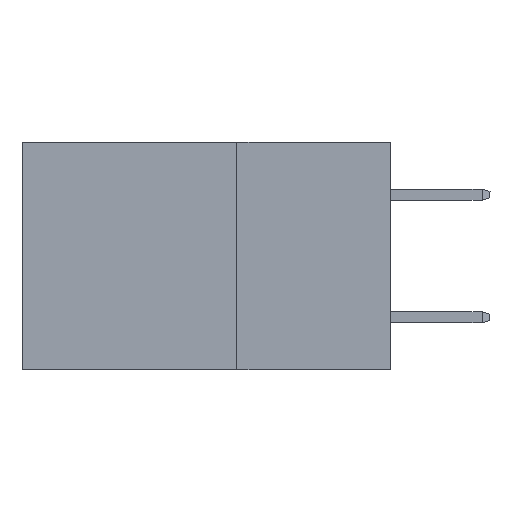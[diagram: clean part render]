
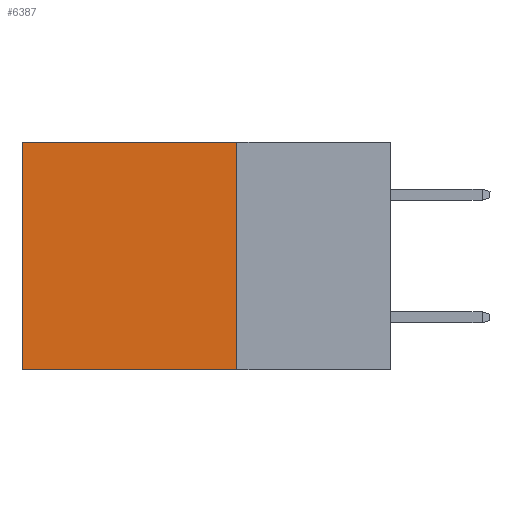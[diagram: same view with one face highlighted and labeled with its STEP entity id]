
A CAD part, left-side view. The second image highlights one B-rep face of the part: STEP entity #6387.
In plain terms, the highlighted planar face has unit normal (-1, 0, 0).
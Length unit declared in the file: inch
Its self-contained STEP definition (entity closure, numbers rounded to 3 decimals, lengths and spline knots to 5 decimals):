
#381 = CARTESIAN_POINT ( 'NONE',  ( 0.2875, 0.25, -0.37 ) ) ;
#484 = EDGE_CURVE ( 'NONE', #5488, #2101, #5989, .T. ) ;
#674 = EDGE_CURVE ( 'NONE', #6831, #8876, #8755, .T. ) ;
#713 = ORIENTED_EDGE ( 'NONE', *, *, #674, .F. ) ;
#784 = LINE ( 'NONE', #3732, #4595 ) ;
#889 = CARTESIAN_POINT ( 'NONE',  ( 0.2875, 0.6, 0. ) ) ;
#1172 = VECTOR ( 'NONE', #2337, 39.37008 ) ;
#1400 = DIRECTION ( 'NONE',  ( 1., 0., 0. ) ) ;
#2101 = VERTEX_POINT ( 'NONE', #5605 ) ;
#2304 = CARTESIAN_POINT ( 'NONE',  ( 0.2875, 0.25, 0. ) ) ;
#2337 = DIRECTION ( 'NONE',  ( 0., 1., 0. ) ) ;
#3276 = EDGE_CURVE ( 'NONE', #8876, #2101, #784, .T. ) ;
#3627 = ORIENTED_EDGE ( 'NONE', *, *, #9447, .T. ) ;
#3655 = AXIS2_PLACEMENT_3D ( 'NONE', #8772, #1400, #7296 ) ;
#3693 = VECTOR ( 'NONE', #9466, 39.37008 ) ;
#3696 = ORIENTED_EDGE ( 'NONE', *, *, #3276, .F. ) ;
#3732 = CARTESIAN_POINT ( 'NONE',  ( 0.2875, 0.25, -0.37 ) ) ;
#4595 = VECTOR ( 'NONE', #7169, 39.37008 ) ;
#5364 = EDGE_LOOP ( 'NONE', ( #9098, #3696, #713, #3627 ) ) ;
#5394 = CARTESIAN_POINT ( 'NONE',  ( 0.2875, 0.25, 0. ) ) ;
#5488 = VERTEX_POINT ( 'NONE', #889 ) ;
#5552 = PLANE ( 'NONE',  #3655 ) ;
#5605 = CARTESIAN_POINT ( 'NONE',  ( 0.2875, 0.6, -0.37 ) ) ;
#5989 = LINE ( 'NONE', #8929, #3693 ) ;
#6387 = ADVANCED_FACE ( 'NONE', ( #8914 ), #5552, .F. ) ;
#6831 = VERTEX_POINT ( 'NONE', #5394 ) ;
#6951 = VECTOR ( 'NONE', #7035, 39.37008 ) ;
#7035 = DIRECTION ( 'NONE',  ( 0., 0., -1. ) ) ;
#7169 = DIRECTION ( 'NONE',  ( 0., 1., 0. ) ) ;
#7296 = DIRECTION ( 'NONE',  ( 0., 0., -1. ) ) ;
#7798 = LINE ( 'NONE', #2304, #1172 ) ;
#8755 = LINE ( 'NONE', #8846, #6951 ) ;
#8772 = CARTESIAN_POINT ( 'NONE',  ( 0.2875, 0.25, 0. ) ) ;
#8846 = CARTESIAN_POINT ( 'NONE',  ( 0.2875, 0.25, 0. ) ) ;
#8876 = VERTEX_POINT ( 'NONE', #381 ) ;
#8914 = FACE_OUTER_BOUND ( 'NONE', #5364, .T. ) ;
#8929 = CARTESIAN_POINT ( 'NONE',  ( 0.2875, 0.6, 0. ) ) ;
#9098 = ORIENTED_EDGE ( 'NONE', *, *, #484, .T. ) ;
#9447 = EDGE_CURVE ( 'NONE', #6831, #5488, #7798, .T. ) ;
#9466 = DIRECTION ( 'NONE',  ( 0., 0., -1. ) ) ;
